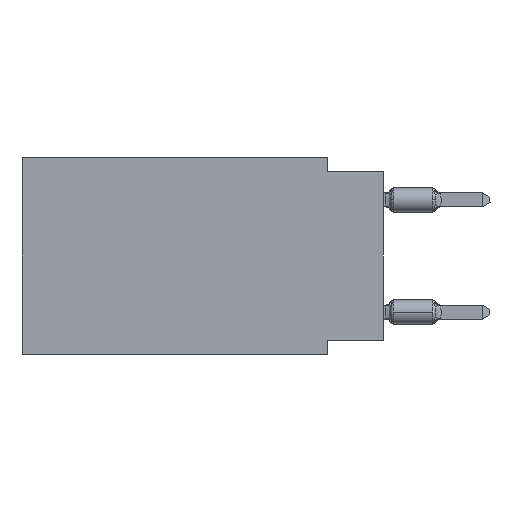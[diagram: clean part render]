
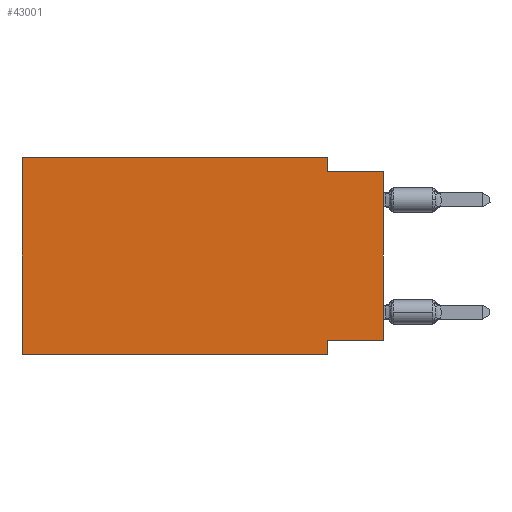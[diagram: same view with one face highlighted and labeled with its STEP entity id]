
A CAD part, left-side view. The second image highlights one B-rep face of the part: STEP entity #43001.
In plain terms, the highlighted planar face has unit normal (-1, 0, 0).
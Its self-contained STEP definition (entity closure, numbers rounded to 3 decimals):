
#753 = LINE ( 'NONE', #28220, #39043 ) ;
#827 = CARTESIAN_POINT ( 'NONE',  ( 0., 0., -8.255 ) ) ;
#1462 = LINE ( 'NONE', #35767, #40719 ) ;
#1494 = CARTESIAN_POINT ( 'NONE',  ( 0., 2.54, -8.89 ) ) ;
#3030 = CARTESIAN_POINT ( 'NONE',  ( 0., 2.54, -8.255 ) ) ;
#3529 = VECTOR ( 'NONE', #27176, 1000. ) ;
#4825 = VERTEX_POINT ( 'NONE', #28611 ) ;
#5614 = EDGE_CURVE ( 'NONE', #24398, #21619, #7612, .T. ) ;
#5652 = CARTESIAN_POINT ( 'NONE',  ( 0., 0., -0.635 ) ) ;
#7612 = LINE ( 'NONE', #38946, #10875 ) ;
#7795 = VECTOR ( 'NONE', #19859, 1000. ) ;
#9023 = FACE_OUTER_BOUND ( 'NONE', #22474, .T. ) ;
#9474 = CARTESIAN_POINT ( 'NONE',  ( 0., 16.383, 0. ) ) ;
#9803 = EDGE_CURVE ( 'NONE', #42642, #43415, #19911, .T. ) ;
#10875 = VECTOR ( 'NONE', #28456, 1000. ) ;
#10908 = CARTESIAN_POINT ( 'NONE',  ( 0., 16.383, -8.89 ) ) ;
#11157 = ORIENTED_EDGE ( 'NONE', *, *, #30619, .F. ) ;
#12680 = DIRECTION ( 'NONE',  ( 0., 0., -1. ) ) ;
#12833 = EDGE_CURVE ( 'NONE', #19142, #25671, #44326, .T. ) ;
#12968 = DIRECTION ( 'NONE',  ( 0., -1., 0. ) ) ;
#13505 = DIRECTION ( 'NONE',  ( 0., 0., -1. ) ) ;
#15892 = EDGE_CURVE ( 'NONE', #43415, #21619, #44286, .T. ) ;
#16251 = CARTESIAN_POINT ( 'NONE',  ( 0., 2.54, 0. ) ) ;
#16331 = PLANE ( 'NONE',  #33897 ) ;
#17375 = CARTESIAN_POINT ( 'NONE',  ( 0., 16.383, 0. ) ) ;
#19142 = VERTEX_POINT ( 'NONE', #3030 ) ;
#19478 = DIRECTION ( 'NONE',  ( 0., -1., 0. ) ) ;
#19672 = ORIENTED_EDGE ( 'NONE', *, *, #37146, .F. ) ;
#19679 = ORIENTED_EDGE ( 'NONE', *, *, #5614, .T. ) ;
#19698 = CARTESIAN_POINT ( 'NONE',  ( 0., 16.383, -8.89 ) ) ;
#19859 = DIRECTION ( 'NONE',  ( 0., -1., 0. ) ) ;
#19911 = LINE ( 'NONE', #16251, #25110 ) ;
#20937 = ORIENTED_EDGE ( 'NONE', *, *, #26714, .F. ) ;
#20941 = VECTOR ( 'NONE', #19478, 1000. ) ;
#21619 = VERTEX_POINT ( 'NONE', #44316 ) ;
#22427 = ORIENTED_EDGE ( 'NONE', *, *, #34062, .T. ) ;
#22474 = EDGE_LOOP ( 'NONE', ( #19679, #31841, #31071, #20937, #19672, #22427, #24550, #11157 ) ) ;
#23429 = DIRECTION ( 'NONE',  ( 1., 0., 0. ) ) ;
#24398 = VERTEX_POINT ( 'NONE', #827 ) ;
#24550 = ORIENTED_EDGE ( 'NONE', *, *, #12833, .F. ) ;
#25110 = VECTOR ( 'NONE', #13505, 1000. ) ;
#25671 = VERTEX_POINT ( 'NONE', #1494 ) ;
#25707 = DIRECTION ( 'NONE',  ( 0., 0., 1. ) ) ;
#26585 = CARTESIAN_POINT ( 'NONE',  ( 0., 2.54, 0. ) ) ;
#26714 = EDGE_CURVE ( 'NONE', #4825, #42642, #37717, .T. ) ;
#26727 = CARTESIAN_POINT ( 'NONE',  ( 0., 2.54, -8.89 ) ) ;
#27176 = DIRECTION ( 'NONE',  ( 0., 0., -1. ) ) ;
#27510 = VERTEX_POINT ( 'NONE', #10908 ) ;
#28220 = CARTESIAN_POINT ( 'NONE',  ( 0., 0., -8.255 ) ) ;
#28456 = DIRECTION ( 'NONE',  ( 0., 0., 1. ) ) ;
#28611 = CARTESIAN_POINT ( 'NONE',  ( 0., 16.383, 0. ) ) ;
#30619 = EDGE_CURVE ( 'NONE', #24398, #19142, #753, .T. ) ;
#31071 = ORIENTED_EDGE ( 'NONE', *, *, #9803, .F. ) ;
#31841 = ORIENTED_EDGE ( 'NONE', *, *, #15892, .F. ) ;
#31875 = DIRECTION ( 'NONE',  ( 0., 1., 0. ) ) ;
#33655 = LINE ( 'NONE', #19698, #20941 ) ;
#33897 = AXIS2_PLACEMENT_3D ( 'NONE', #9474, #23429, #12680 ) ;
#34062 = EDGE_CURVE ( 'NONE', #27510, #25671, #33655, .T. ) ;
#35767 = CARTESIAN_POINT ( 'NONE',  ( 0., 16.383, 0. ) ) ;
#37146 = EDGE_CURVE ( 'NONE', #27510, #4825, #1462, .T. ) ;
#37717 = LINE ( 'NONE', #17375, #7795 ) ;
#38946 = CARTESIAN_POINT ( 'NONE',  ( 0., 0., 0. ) ) ;
#39043 = VECTOR ( 'NONE', #31875, 1000. ) ;
#40719 = VECTOR ( 'NONE', #25707, 1000. ) ;
#40945 = VECTOR ( 'NONE', #12968, 1000. ) ;
#42642 = VERTEX_POINT ( 'NONE', #26585 ) ;
#42775 = CARTESIAN_POINT ( 'NONE',  ( 0., 2.54, -0.635 ) ) ;
#43001 = ADVANCED_FACE ( 'NONE', ( #9023 ), #16331, .F. ) ;
#43415 = VERTEX_POINT ( 'NONE', #42775 ) ;
#44286 = LINE ( 'NONE', #5652, #40945 ) ;
#44316 = CARTESIAN_POINT ( 'NONE',  ( 0., 0., -0.635 ) ) ;
#44326 = LINE ( 'NONE', #26727, #3529 ) ;
